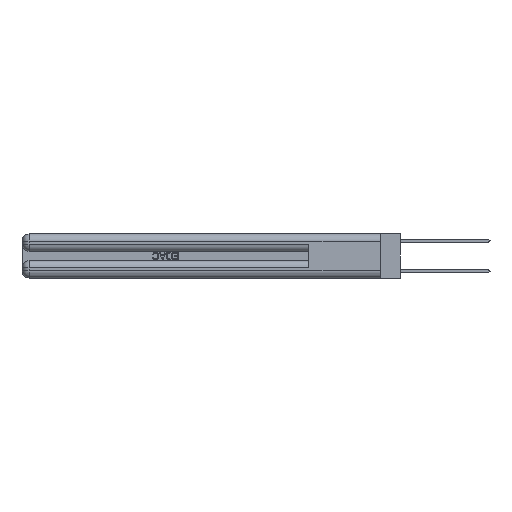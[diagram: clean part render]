
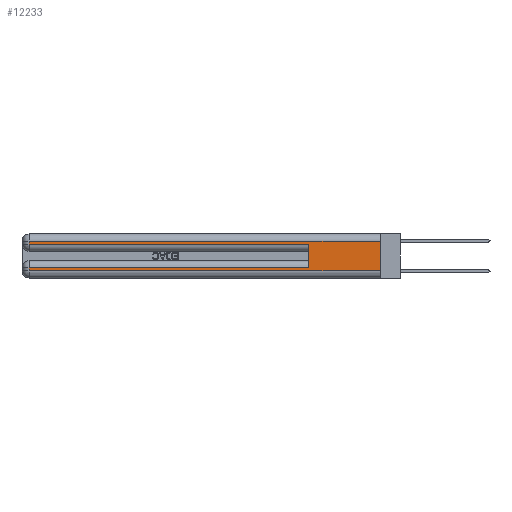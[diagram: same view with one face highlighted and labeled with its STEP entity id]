
A CAD part, left-side view. The second image highlights one B-rep face of the part: STEP entity #12233.
In plain terms, the highlighted planar face has unit normal (-1, 0, 0).
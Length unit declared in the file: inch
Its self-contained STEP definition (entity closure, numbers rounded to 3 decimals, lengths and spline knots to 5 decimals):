
#215 = CARTESIAN_POINT ( 'NONE',  ( 0., 0.6, 0.145 ) ) ;
#246 = LINE ( 'NONE', #29445, #26752 ) ;
#909 = LINE ( 'NONE', #13435, #6961 ) ;
#2114 = CARTESIAN_POINT ( 'NONE',  ( 0., 2.94, 0.06 ) ) ;
#2191 = EDGE_CURVE ( 'NONE', #27573, #25671, #6870, .T. ) ;
#2219 = VERTEX_POINT ( 'NONE', #9661 ) ;
#2812 = DIRECTION ( 'NONE',  ( 0., 0., 1. ) ) ;
#3297 = VECTOR ( 'NONE', #18669, 39.37008 ) ;
#3659 = LINE ( 'NONE', #215, #16556 ) ;
#3832 = VERTEX_POINT ( 'NONE', #9217 ) ;
#4319 = DIRECTION ( 'NONE',  ( 0., 1., 0. ) ) ;
#4469 = ORIENTED_EDGE ( 'NONE', *, *, #15341, .T. ) ;
#5111 = ORIENTED_EDGE ( 'NONE', *, *, #19434, .T. ) ;
#5228 = CARTESIAN_POINT ( 'NONE',  ( 0., 0., 0.06 ) ) ;
#6584 = CARTESIAN_POINT ( 'NONE',  ( 0., 2.94, 0.37 ) ) ;
#6870 = LINE ( 'NONE', #12110, #25710 ) ;
#6961 = VECTOR ( 'NONE', #21150, 39.37008 ) ;
#6979 = PLANE ( 'NONE',  #11508 ) ;
#7136 = EDGE_CURVE ( 'NONE', #3832, #2219, #16925, .T. ) ;
#7929 = FACE_OUTER_BOUND ( 'NONE', #14902, .T. ) ;
#8352 = ORIENTED_EDGE ( 'NONE', *, *, #15939, .F. ) ;
#8490 = VECTOR ( 'NONE', #16355, 39.37008 ) ;
#9201 = DIRECTION ( 'NONE',  ( 0., 0., -1. ) ) ;
#9217 = CARTESIAN_POINT ( 'NONE',  ( 0., 0., 0.31 ) ) ;
#9567 = CARTESIAN_POINT ( 'NONE',  ( 0., 0.6, 0.285 ) ) ;
#9584 = CARTESIAN_POINT ( 'NONE',  ( 0., 0., 0.37 ) ) ;
#9661 = CARTESIAN_POINT ( 'NONE',  ( 0., 0., 0.06 ) ) ;
#11490 = LINE ( 'NONE', #6584, #24299 ) ;
#11508 = AXIS2_PLACEMENT_3D ( 'NONE', #9584, #27484, #12138 ) ;
#11680 = VECTOR ( 'NONE', #20606, 39.37008 ) ;
#11767 = ORIENTED_EDGE ( 'NONE', *, *, #26750, .T. ) ;
#12110 = CARTESIAN_POINT ( 'NONE',  ( 0., 0., 0.085 ) ) ;
#12138 = DIRECTION ( 'NONE',  ( 0., 0., -1. ) ) ;
#12233 = ADVANCED_FACE ( 'NONE', ( #7929 ), #6979, .F. ) ;
#12793 = EDGE_CURVE ( 'NONE', #25671, #16459, #11490, .T. ) ;
#13435 = CARTESIAN_POINT ( 'NONE',  ( 0., 0., 0.31 ) ) ;
#14454 = VERTEX_POINT ( 'NONE', #9567 ) ;
#14902 = EDGE_LOOP ( 'NONE', ( #27913, #4469, #5111, #23730, #8352, #24375, #25414, #11767 ) ) ;
#15341 = EDGE_CURVE ( 'NONE', #3832, #22533, #909, .T. ) ;
#15781 = CARTESIAN_POINT ( 'NONE',  ( 0., 2.94, 0.31 ) ) ;
#15939 = EDGE_CURVE ( 'NONE', #27573, #14454, #3659, .T. ) ;
#16108 = CARTESIAN_POINT ( 'NONE',  ( 0., 2.94, 0.37 ) ) ;
#16197 = LINE ( 'NONE', #16108, #3297 ) ;
#16355 = DIRECTION ( 'NONE',  ( 0., 0., -1. ) ) ;
#16459 = VERTEX_POINT ( 'NONE', #2114 ) ;
#16556 = VECTOR ( 'NONE', #2812, 39.37008 ) ;
#16698 = DIRECTION ( 'NONE',  ( 0., -1., 0. ) ) ;
#16925 = LINE ( 'NONE', #29105, #8490 ) ;
#17236 = VERTEX_POINT ( 'NONE', #24945 ) ;
#18442 = CARTESIAN_POINT ( 'NONE',  ( 0., 2.94, 0.085 ) ) ;
#18669 = DIRECTION ( 'NONE',  ( 0., 0., -1. ) ) ;
#19434 = EDGE_CURVE ( 'NONE', #22533, #17236, #16197, .T. ) ;
#20606 = DIRECTION ( 'NONE',  ( 0., -1., 0. ) ) ;
#21150 = DIRECTION ( 'NONE',  ( 0., 1., 0. ) ) ;
#22533 = VERTEX_POINT ( 'NONE', #15781 ) ;
#23730 = ORIENTED_EDGE ( 'NONE', *, *, #30914, .T. ) ;
#24299 = VECTOR ( 'NONE', #9201, 39.37008 ) ;
#24375 = ORIENTED_EDGE ( 'NONE', *, *, #2191, .T. ) ;
#24945 = CARTESIAN_POINT ( 'NONE',  ( 0., 2.94, 0.285 ) ) ;
#25414 = ORIENTED_EDGE ( 'NONE', *, *, #12793, .T. ) ;
#25671 = VERTEX_POINT ( 'NONE', #18442 ) ;
#25710 = VECTOR ( 'NONE', #4319, 39.37008 ) ;
#26750 = EDGE_CURVE ( 'NONE', #16459, #2219, #32159, .T. ) ;
#26752 = VECTOR ( 'NONE', #16698, 39.37008 ) ;
#27484 = DIRECTION ( 'NONE',  ( 1., 0., 0. ) ) ;
#27573 = VERTEX_POINT ( 'NONE', #31566 ) ;
#27913 = ORIENTED_EDGE ( 'NONE', *, *, #7136, .F. ) ;
#29105 = CARTESIAN_POINT ( 'NONE',  ( 0., 0., 0.37 ) ) ;
#29445 = CARTESIAN_POINT ( 'NONE',  ( 0., 0., 0.285 ) ) ;
#30914 = EDGE_CURVE ( 'NONE', #17236, #14454, #246, .T. ) ;
#31566 = CARTESIAN_POINT ( 'NONE',  ( 0., 0.6, 0.085 ) ) ;
#32159 = LINE ( 'NONE', #5228, #11680 ) ;
